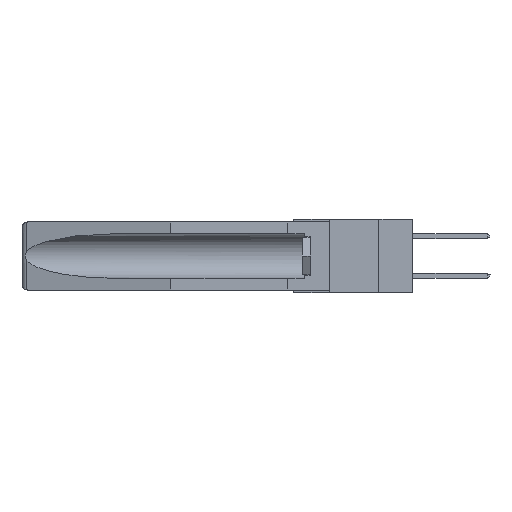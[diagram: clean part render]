
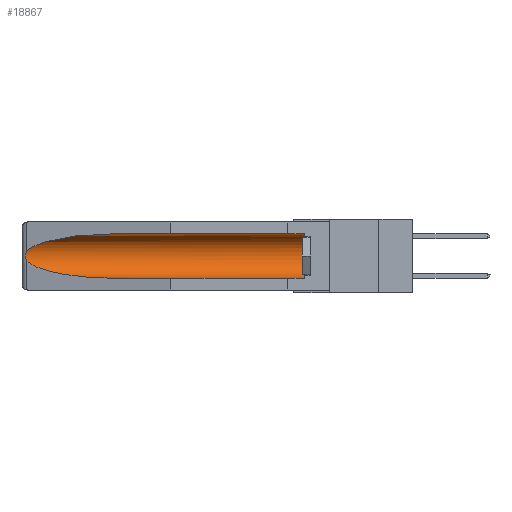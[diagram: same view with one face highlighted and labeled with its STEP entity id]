
A CAD part, left-side view. The second image highlights one B-rep face of the part: STEP entity #18867.
In plain terms, the highlighted cylindrical face has radius 2.857 mm (diameter 5.715 mm), a partial arc.
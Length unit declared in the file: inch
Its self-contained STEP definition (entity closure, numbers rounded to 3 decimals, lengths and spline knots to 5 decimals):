
#2582 = VERTEX_POINT ( 'NONE', #7479 ) ;
#2678 = VERTEX_POINT ( 'NONE', #5675 ) ;
#2921 = LINE ( 'NONE', #10896, #25559 ) ;
#2946 = CARTESIAN_POINT ( 'NONE',  ( 0.26537, 1.52718, -0.19328 ) ) ;
#3568 = CARTESIAN_POINT ( 'NONE',  ( 0.2673, 1.5327, -0.16383 ) ) ;
#4686 = CARTESIAN_POINT ( 'NONE',  ( 0.155, 1.07973, -0.059 ) ) ;
#4916 = EDGE_CURVE ( 'NONE', #21912, #20359, #23176, .T. ) ;
#5064 = FACE_OUTER_BOUND ( 'NONE', #7156, .T. ) ;
#5583 = CARTESIAN_POINT ( 'NONE',  ( 0.155, -0.30754, -0.059 ) ) ;
#5675 = CARTESIAN_POINT ( 'NONE',  ( 0.155, 0.126, -0.059 ) ) ;
#5867 = CARTESIAN_POINT ( 'NONE',  ( 0.26654, 1.53092, -0.15636 ) ) ;
#7156 = EDGE_LOOP ( 'NONE', ( #14209, #14617, #20379, #21435, #14489, #26143 ) ) ;
#7308 = CARTESIAN_POINT ( 'NONE',  ( 0.155, 1.07973, -0.059 ) ) ;
#7479 = CARTESIAN_POINT ( 'NONE',  ( 0.155, 0.126, -0.284 ) ) ;
#8240 = CARTESIAN_POINT ( 'NONE',  ( 0.21114, 1.30732, -0.284 ) ) ;
#8287 = DIRECTION ( 'NONE',  ( 0., 0., 1. ) ) ;
#8329 = CARTESIAN_POINT ( 'NONE',  ( 0.26537, 1.52718, -0.19328 ) ) ;
#8955 =( BOUNDED_CURVE ( )  B_SPLINE_CURVE ( 3, ( #7308, #20339, #13524, #24223 ),
 .UNSPECIFIED., .F., .F. ) 
 B_SPLINE_CURVE_WITH_KNOTS ( ( 4, 4 ),
 ( 4.71239, 6.08839 ),
 .UNSPECIFIED. ) 
 CURVE ( )  GEOMETRIC_REPRESENTATION_ITEM ( )  RATIONAL_B_SPLINE_CURVE ( ( 1., 0.848, 0.848, 1. ) ) 
 REPRESENTATION_ITEM ( '' )  );
#10080 = CARTESIAN_POINT ( 'NONE',  ( 0.26537, 1.52718, -0.14972 ) ) ;
#10761 = CARTESIAN_POINT ( 'NONE',  ( 0.25451, 1.48313, -0.24835 ) ) ;
#10896 = CARTESIAN_POINT ( 'NONE',  ( 0.155, -0.30754, -0.284 ) ) ;
#11260 = CIRCLE ( 'NONE', #21840, 0.1125 ) ;
#12046 = DIRECTION ( 'NONE',  ( 0., -1., 0. ) ) ;
#12135 = DIRECTION ( 'NONE',  ( 0., 0., 1. ) ) ;
#12172 = VECTOR ( 'NONE', #18124, 39.37008 ) ;
#12256 = CARTESIAN_POINT ( 'NONE',  ( 0.2673, 1.53269, -0.17917 ) ) ;
#12490 = EDGE_CURVE ( 'NONE', #25670, #21912, #8955, .T. ) ;
#12669 = CARTESIAN_POINT ( 'NONE',  ( 0.155, 1.07973, -0.284 ) ) ;
#12887 = CARTESIAN_POINT ( 'NONE',  ( 0.155, 1.07973, -0.284 ) ) ;
#13524 = CARTESIAN_POINT ( 'NONE',  ( 0.25451, 1.48313, -0.09465 ) ) ;
#13945 = EDGE_CURVE ( 'NONE', #2582, #24139, #2921, .T. ) ;
#13950 = AXIS2_PLACEMENT_3D ( 'NONE', #26934, #20493, #8287 ) ;
#14209 = ORIENTED_EDGE ( 'NONE', *, *, #12490, .T. ) ;
#14239 = EDGE_CURVE ( 'NONE', #20359, #24139, #25593, .T. ) ;
#14489 = ORIENTED_EDGE ( 'NONE', *, *, #16050, .T. ) ;
#14617 = ORIENTED_EDGE ( 'NONE', *, *, #4916, .T. ) ;
#16050 = EDGE_CURVE ( 'NONE', #2582, #2678, #11260, .T. ) ;
#16497 = CYLINDRICAL_SURFACE ( 'NONE', #13950, 0.1125 ) ;
#16501 = CARTESIAN_POINT ( 'NONE',  ( 0.26655, 1.53094, -0.18657 ) ) ;
#16571 = LINE ( 'NONE', #5583, #12172 ) ;
#16758 = CARTESIAN_POINT ( 'NONE',  ( 0.155, 0.126, -0.1715 ) ) ;
#18124 = DIRECTION ( 'NONE',  ( 0., 1., 0. ) ) ;
#18599 = CARTESIAN_POINT ( 'NONE',  ( 0.26537, 1.52718, -0.14972 ) ) ;
#18785 = CARTESIAN_POINT ( 'NONE',  ( 0.2675, 1.53308, -0.17534 ) ) ;
#18867 = ADVANCED_FACE ( 'NONE', ( #5064 ), #16497, .F. ) ;
#18876 = CARTESIAN_POINT ( 'NONE',  ( 0.26597, 1.52961, -0.15275 ) ) ;
#20339 = CARTESIAN_POINT ( 'NONE',  ( 0.21114, 1.30732, -0.059 ) ) ;
#20359 = VERTEX_POINT ( 'NONE', #2946 ) ;
#20379 = ORIENTED_EDGE ( 'NONE', *, *, #14239, .T. ) ;
#20493 = DIRECTION ( 'NONE',  ( 0., 1., 0. ) ) ;
#20942 = CARTESIAN_POINT ( 'NONE',  ( 0.2675, 1.53308, -0.16763 ) ) ;
#21048 = CARTESIAN_POINT ( 'NONE',  ( 0.26537, 1.52718, -0.19328 ) ) ;
#21435 = ORIENTED_EDGE ( 'NONE', *, *, #13945, .F. ) ;
#21840 = AXIS2_PLACEMENT_3D ( 'NONE', #16758, #12046, #12135 ) ;
#21912 = VERTEX_POINT ( 'NONE', #18599 ) ;
#22654 = EDGE_CURVE ( 'NONE', #2678, #25670, #16571, .T. ) ;
#23176 = B_SPLINE_CURVE_WITH_KNOTS ( 'NONE', 3,
 ( #10080, #18876, #5867, #3568, #20942, #18785, #12256, #16501, #25212, #21048 ),
 .UNSPECIFIED., .F., .F.,
 ( 4, 2, 2, 2, 4 ),
 ( 0., 0.00029, 0.00058, 0.00087, 0.00117 ),
 .UNSPECIFIED. ) ;
#23937 = DIRECTION ( 'NONE',  ( 0., 1., 0. ) ) ;
#24139 = VERTEX_POINT ( 'NONE', #12887 ) ;
#24223 = CARTESIAN_POINT ( 'NONE',  ( 0.26537, 1.52718, -0.14972 ) ) ;
#25212 = CARTESIAN_POINT ( 'NONE',  ( 0.26597, 1.5296, -0.19026 ) ) ;
#25559 = VECTOR ( 'NONE', #23937, 39.37008 ) ;
#25593 =( BOUNDED_CURVE ( )  B_SPLINE_CURVE ( 3, ( #8329, #10761, #8240, #12669 ),
 .UNSPECIFIED., .F., .F. ) 
 B_SPLINE_CURVE_WITH_KNOTS ( ( 4, 4 ),
 ( 0.1948, 1.5708 ),
 .UNSPECIFIED. ) 
 CURVE ( )  GEOMETRIC_REPRESENTATION_ITEM ( )  RATIONAL_B_SPLINE_CURVE ( ( 1., 0.848, 0.848, 1. ) ) 
 REPRESENTATION_ITEM ( '' )  );
#25670 = VERTEX_POINT ( 'NONE', #4686 ) ;
#26143 = ORIENTED_EDGE ( 'NONE', *, *, #22654, .T. ) ;
#26934 = CARTESIAN_POINT ( 'NONE',  ( 0.155, -0.30754, -0.1715 ) ) ;
